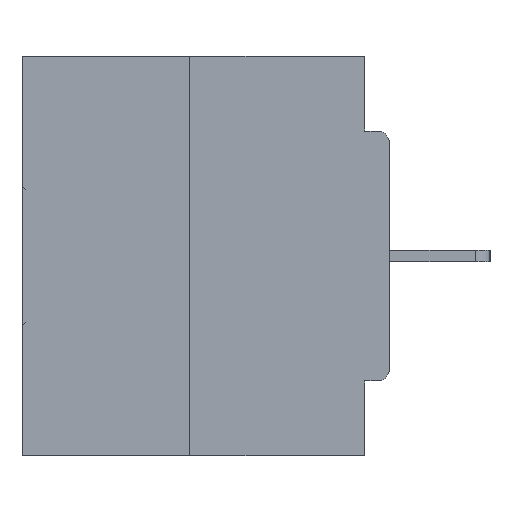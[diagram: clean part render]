
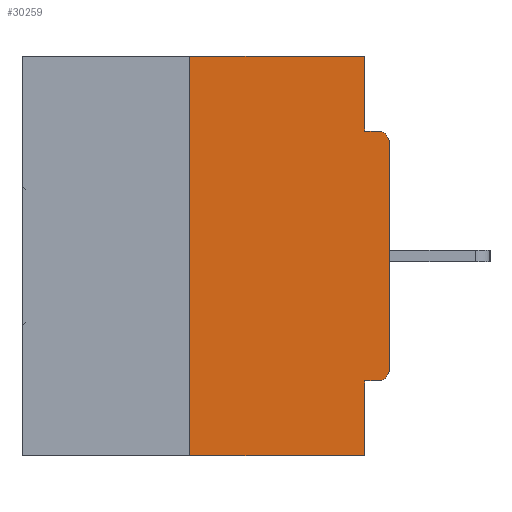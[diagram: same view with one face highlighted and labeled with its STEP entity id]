
A CAD part, left-side view. The second image highlights one B-rep face of the part: STEP entity #30259.
In plain terms, the highlighted planar face has unit normal (-1, 0, 0).
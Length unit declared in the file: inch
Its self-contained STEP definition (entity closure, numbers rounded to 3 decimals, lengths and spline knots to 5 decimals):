
#190 = VERTEX_POINT ( 'NONE', #36272 ) ;
#481 = LINE ( 'NONE', #11494, #22759 ) ;
#1446 = AXIS2_PLACEMENT_3D ( 'NONE', #30622, #5442, #5794 ) ;
#1586 = ORIENTED_EDGE ( 'NONE', *, *, #23014, .F. ) ;
#1889 = LINE ( 'NONE', #26855, #5169 ) ;
#2740 = EDGE_CURVE ( 'NONE', #19250, #190, #481, .T. ) ;
#3829 = ORIENTED_EDGE ( 'NONE', *, *, #2740, .F. ) ;
#4850 = LINE ( 'NONE', #27810, #21211 ) ;
#5169 = VECTOR ( 'NONE', #24463, 39.37008 ) ;
#5403 = CARTESIAN_POINT ( 'NONE',  ( 0., 0.031, 0. ) ) ;
#5442 = DIRECTION ( 'NONE',  ( 1., 0., 0. ) ) ;
#5692 = ORIENTED_EDGE ( 'NONE', *, *, #28621, .F. ) ;
#5794 = DIRECTION ( 'NONE',  ( 0., 0., -1. ) ) ;
#6207 = CARTESIAN_POINT ( 'NONE',  ( 0., 0.25, -0.5 ) ) ;
#6340 = EDGE_CURVE ( 'NONE', #14465, #23998, #19282, .T. ) ;
#6798 = AXIS2_PLACEMENT_3D ( 'NONE', #18081, #14979, #26378 ) ;
#7599 = ORIENTED_EDGE ( 'NONE', *, *, #18649, .F. ) ;
#8724 = CARTESIAN_POINT ( 'NONE',  ( 0., 0., 0. ) ) ;
#8746 = CARTESIAN_POINT ( 'NONE',  ( 0., 0.25, 0. ) ) ;
#8749 = EDGE_CURVE ( 'NONE', #31297, #14465, #22679, .T. ) ;
#11494 = CARTESIAN_POINT ( 'NONE',  ( 0., 0.031, -0.5 ) ) ;
#11639 = VECTOR ( 'NONE', #22034, 39.37008 ) ;
#11654 = VERTEX_POINT ( 'NONE', #5403 ) ;
#12487 = VERTEX_POINT ( 'NONE', #35627 ) ;
#12724 = CARTESIAN_POINT ( 'NONE',  ( 0., 0.031, 0. ) ) ;
#13177 = CARTESIAN_POINT ( 'NONE',  ( 0., 0.46, 0. ) ) ;
#13275 = DIRECTION ( 'NONE',  ( 0., 0., -1. ) ) ;
#13320 = LINE ( 'NONE', #30624, #16378 ) ;
#13580 = VERTEX_POINT ( 'NONE', #15420 ) ;
#13804 = CARTESIAN_POINT ( 'NONE',  ( 0., 0., -0.1085 ) ) ;
#14465 = VERTEX_POINT ( 'NONE', #13804 ) ;
#14979 = DIRECTION ( 'NONE',  ( -1., 0., 0. ) ) ;
#15039 = CARTESIAN_POINT ( 'NONE',  ( 0., 0.015, -0.1085 ) ) ;
#15214 = DIRECTION ( 'NONE',  ( 0., 0., -1. ) ) ;
#15319 = VERTEX_POINT ( 'NONE', #8746 ) ;
#15420 = CARTESIAN_POINT ( 'NONE',  ( 0., 0.015, -0.4065 ) ) ;
#16047 = DIRECTION ( 'NONE',  ( 0., 1., 0. ) ) ;
#16378 = VECTOR ( 'NONE', #24538, 39.37008 ) ;
#17897 = ORIENTED_EDGE ( 'NONE', *, *, #18173, .T. ) ;
#17940 = ORIENTED_EDGE ( 'NONE', *, *, #31751, .T. ) ;
#18081 = CARTESIAN_POINT ( 'NONE',  ( 0., 0.015, -0.3915 ) ) ;
#18173 = EDGE_CURVE ( 'NONE', #21065, #190, #1889, .T. ) ;
#18649 = EDGE_CURVE ( 'NONE', #12487, #23998, #32711, .T. ) ;
#18963 = LINE ( 'NONE', #12724, #30126 ) ;
#19002 = VECTOR ( 'NONE', #30287, 39.37008 ) ;
#19250 = VERTEX_POINT ( 'NONE', #22710 ) ;
#19282 = CIRCLE ( 'NONE', #35721, 0.015 ) ;
#19318 = CARTESIAN_POINT ( 'NONE',  ( 0., 0.015, -0.0935 ) ) ;
#19915 = DIRECTION ( 'NONE',  ( 0., 0., 1. ) ) ;
#20424 = EDGE_LOOP ( 'NONE', ( #5692, #27678, #17897, #3829, #1586, #17940, #31163, #24279, #7599, #32726 ) ) ;
#20917 = DIRECTION ( 'NONE',  ( -1., 0., 0. ) ) ;
#21065 = VERTEX_POINT ( 'NONE', #6207 ) ;
#21211 = VECTOR ( 'NONE', #16047, 39.37008 ) ;
#21375 = EDGE_CURVE ( 'NONE', #21065, #15319, #13320, .T. ) ;
#22034 = DIRECTION ( 'NONE',  ( 0., -1., 0. ) ) ;
#22679 = LINE ( 'NONE', #8724, #29056 ) ;
#22710 = CARTESIAN_POINT ( 'NONE',  ( 0., 0.031, -0.4065 ) ) ;
#22759 = VECTOR ( 'NONE', #33932, 39.37008 ) ;
#23014 = EDGE_CURVE ( 'NONE', #13580, #19250, #4850, .T. ) ;
#23803 = CIRCLE ( 'NONE', #6798, 0.015 ) ;
#23998 = VERTEX_POINT ( 'NONE', #19318 ) ;
#24279 = ORIENTED_EDGE ( 'NONE', *, *, #6340, .T. ) ;
#24463 = DIRECTION ( 'NONE',  ( 0., -1., 0. ) ) ;
#24538 = DIRECTION ( 'NONE',  ( 0., 0., 1. ) ) ;
#25009 = EDGE_CURVE ( 'NONE', #11654, #12487, #18963, .T. ) ;
#26378 = DIRECTION ( 'NONE',  ( 0., 0., -1. ) ) ;
#26855 = CARTESIAN_POINT ( 'NONE',  ( 0., 0.46, -0.5 ) ) ;
#27678 = ORIENTED_EDGE ( 'NONE', *, *, #21375, .F. ) ;
#27810 = CARTESIAN_POINT ( 'NONE',  ( 0., 0., -0.4065 ) ) ;
#27851 = PLANE ( 'NONE',  #1446 ) ;
#28621 = EDGE_CURVE ( 'NONE', #15319, #11654, #29913, .T. ) ;
#29056 = VECTOR ( 'NONE', #19915, 39.37008 ) ;
#29913 = LINE ( 'NONE', #13177, #19002 ) ;
#29959 = CARTESIAN_POINT ( 'NONE',  ( 0., 0., -0.0935 ) ) ;
#30126 = VECTOR ( 'NONE', #13275, 39.37008 ) ;
#30242 = CARTESIAN_POINT ( 'NONE',  ( 0., 0., -0.3915 ) ) ;
#30259 = ADVANCED_FACE ( 'NONE', ( #33009 ), #27851, .F. ) ;
#30287 = DIRECTION ( 'NONE',  ( 0., -1., 0. ) ) ;
#30622 = CARTESIAN_POINT ( 'NONE',  ( 0., 0.46, 0. ) ) ;
#30624 = CARTESIAN_POINT ( 'NONE',  ( 0., 0.25, 0. ) ) ;
#31163 = ORIENTED_EDGE ( 'NONE', *, *, #8749, .T. ) ;
#31297 = VERTEX_POINT ( 'NONE', #30242 ) ;
#31751 = EDGE_CURVE ( 'NONE', #13580, #31297, #23803, .T. ) ;
#32711 = LINE ( 'NONE', #29959, #11639 ) ;
#32726 = ORIENTED_EDGE ( 'NONE', *, *, #25009, .F. ) ;
#33009 = FACE_OUTER_BOUND ( 'NONE', #20424, .T. ) ;
#33932 = DIRECTION ( 'NONE',  ( 0., 0., -1. ) ) ;
#35627 = CARTESIAN_POINT ( 'NONE',  ( 0., 0.031, -0.0935 ) ) ;
#35721 = AXIS2_PLACEMENT_3D ( 'NONE', #15039, #20917, #15214 ) ;
#36272 = CARTESIAN_POINT ( 'NONE',  ( 0., 0.031, -0.5 ) ) ;
